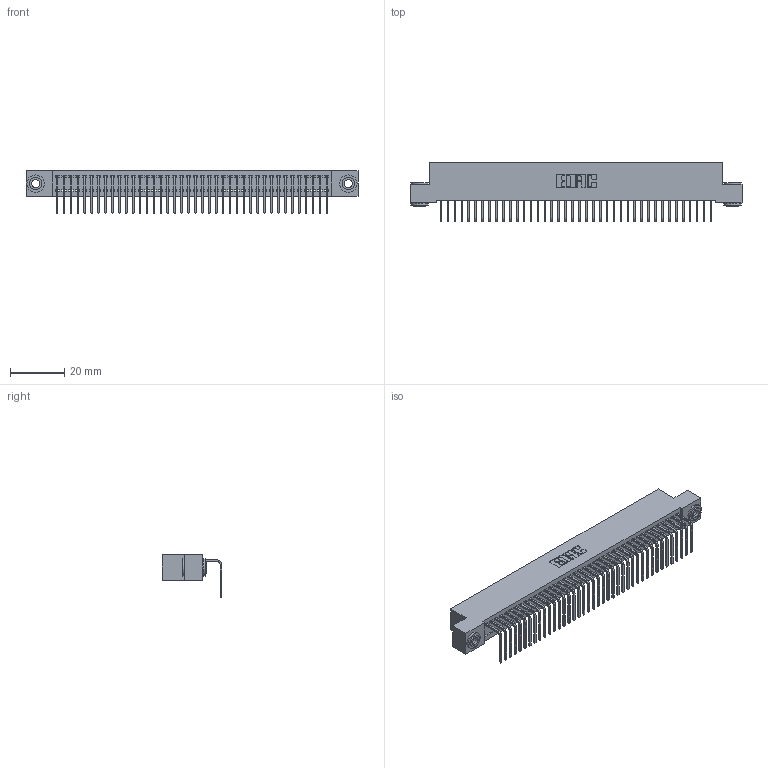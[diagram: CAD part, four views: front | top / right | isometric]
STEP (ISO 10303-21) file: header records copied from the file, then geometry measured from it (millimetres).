
FILE_DESCRIPTION (( 'STEP AP203' ), '1' );
FILE_NAME ('392-040-558-103.STEP', '2018-08-16T12:29:50', ( '' ), ( '' ), 'SwSTEP 2.0', 'SolidWorks 2016', '' );
FILE_SCHEMA (( 'CONFIG_CONTROL_DESIGN' ));
Length unit declared in the file: inch
Products named in the file (4): 345-292-001_558 Tail - 2; 342-250-002_345-250-002-102; 392-040-558-103; 342 Part_.156 TH
Assembly tree (43 placements, depth 2):
  392-040-558-103
    342 Part_.156 TH
    345-292-001_558 Tail - 2  x40
    342-250-002_345-250-002-102  x2
Bounding box: 121.92 x 21.91 x 15.62 mm (x, y, z)
Volume: 10838.7 mm3; surface area: 16861.8 mm2
Topology: 43 solids, 43 shells, 2548 faces, 7655 edges, 5046 vertices
Faces by surface type: plane 1836, cylinder 704, cone 8
Entity records: 25314 total; most frequent: CARTESIAN_POINT 4345, ORIENTED_EDGE 4314, DIRECTION 3703, EDGE_CURVE 2157, VECTOR 2005, LINE 2005, VERTEX_POINT 1434, AXIS2_PLACEMENT_3D 849
